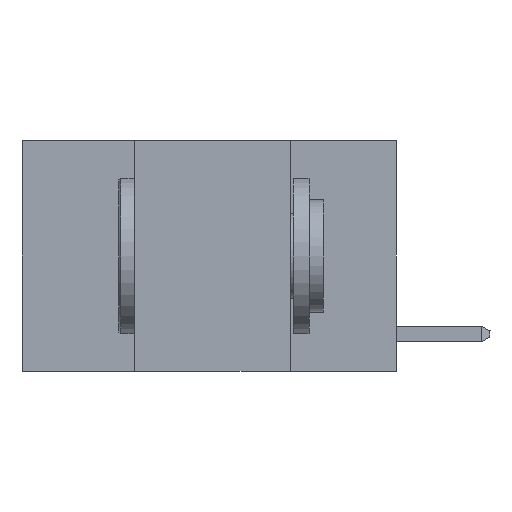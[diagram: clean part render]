
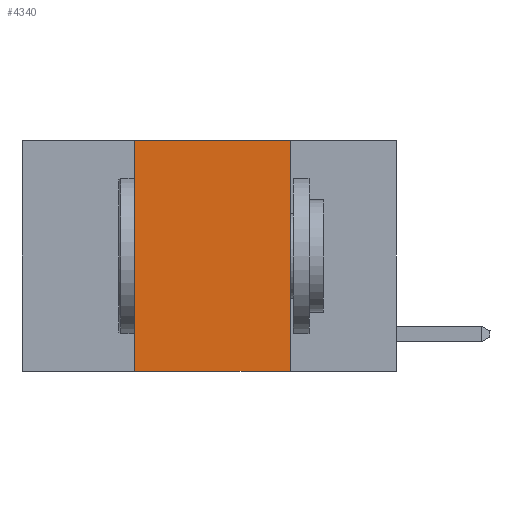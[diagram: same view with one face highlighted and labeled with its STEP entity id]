
A CAD part, left-side view. The second image highlights one B-rep face of the part: STEP entity #4340.
In plain terms, the highlighted planar face has unit normal (-1, 0, 0).
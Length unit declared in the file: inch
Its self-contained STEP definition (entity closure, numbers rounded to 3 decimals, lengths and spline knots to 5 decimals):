
#506 = VERTEX_POINT ( 'NONE', #21758 ) ;
#840 = LINE ( 'NONE', #13297, #24597 ) ;
#850 = LINE ( 'NONE', #1537, #9315 ) ;
#1537 = CARTESIAN_POINT ( 'NONE',  ( 0., 0.42, 0. ) ) ;
#2718 = VECTOR ( 'NONE', #24501, 39.37008 ) ;
#3351 = EDGE_CURVE ( 'NONE', #19554, #12028, #17927, .T. ) ;
#3574 = DIRECTION ( 'NONE',  ( 0., -1., 0. ) ) ;
#3589 = VERTEX_POINT ( 'NONE', #23277 ) ;
#3699 = DIRECTION ( 'NONE',  ( 0., -1., 0. ) ) ;
#3873 = EDGE_LOOP ( 'NONE', ( #8116, #16897, #14653, #4058 ) ) ;
#3991 = EDGE_CURVE ( 'NONE', #3589, #506, #850, .T. ) ;
#4058 = ORIENTED_EDGE ( 'NONE', *, *, #19635, .T. ) ;
#4340 = ADVANCED_FACE ( 'NONE', ( #16703 ), #17732, .F. ) ;
#4503 = DIRECTION ( 'NONE',  ( 1., 0., 0. ) ) ;
#8116 = ORIENTED_EDGE ( 'NONE', *, *, #3351, .F. ) ;
#8284 = CARTESIAN_POINT ( 'NONE',  ( 0., 0.6, 0. ) ) ;
#9135 = CARTESIAN_POINT ( 'NONE',  ( 0., 0.17, 0. ) ) ;
#9315 = VECTOR ( 'NONE', #14935, 39.37008 ) ;
#12028 = VERTEX_POINT ( 'NONE', #17952 ) ;
#12534 = AXIS2_PLACEMENT_3D ( 'NONE', #8284, #4503, #17815 ) ;
#13297 = CARTESIAN_POINT ( 'NONE',  ( 0., 0.6, 0. ) ) ;
#13595 = LINE ( 'NONE', #15019, #18634 ) ;
#14653 = ORIENTED_EDGE ( 'NONE', *, *, #3991, .F. ) ;
#14877 = CARTESIAN_POINT ( 'NONE',  ( 0., 0.17, 0. ) ) ;
#14935 = DIRECTION ( 'NONE',  ( 0., 0., 1. ) ) ;
#15019 = CARTESIAN_POINT ( 'NONE',  ( 0., 0.6, -0.37 ) ) ;
#16703 = FACE_OUTER_BOUND ( 'NONE', #3873, .T. ) ;
#16767 = EDGE_CURVE ( 'NONE', #506, #19554, #840, .T. ) ;
#16897 = ORIENTED_EDGE ( 'NONE', *, *, #16767, .F. ) ;
#17732 = PLANE ( 'NONE',  #12534 ) ;
#17815 = DIRECTION ( 'NONE',  ( 0., 0., -1. ) ) ;
#17927 = LINE ( 'NONE', #14877, #2718 ) ;
#17952 = CARTESIAN_POINT ( 'NONE',  ( 0., 0.17, -0.37 ) ) ;
#18634 = VECTOR ( 'NONE', #3574, 39.37008 ) ;
#19554 = VERTEX_POINT ( 'NONE', #9135 ) ;
#19635 = EDGE_CURVE ( 'NONE', #3589, #12028, #13595, .T. ) ;
#21758 = CARTESIAN_POINT ( 'NONE',  ( 0., 0.42, 0. ) ) ;
#23277 = CARTESIAN_POINT ( 'NONE',  ( 0., 0.42, -0.37 ) ) ;
#24501 = DIRECTION ( 'NONE',  ( 0., 0., -1. ) ) ;
#24597 = VECTOR ( 'NONE', #3699, 39.37008 ) ;
